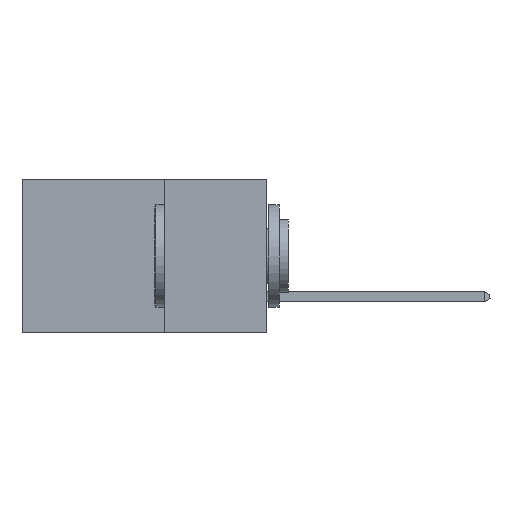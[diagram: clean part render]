
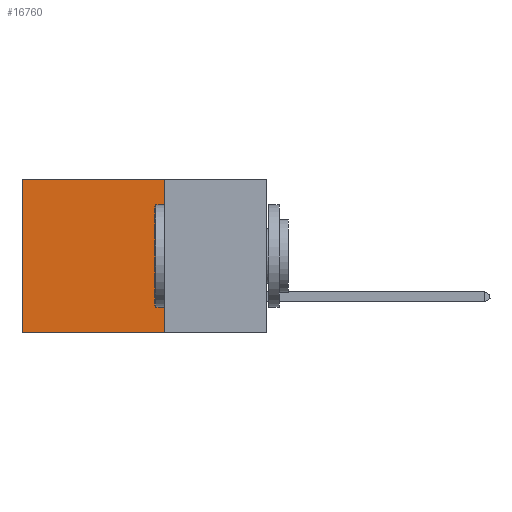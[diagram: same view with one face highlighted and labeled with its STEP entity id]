
A CAD part, left-side view. The second image highlights one B-rep face of the part: STEP entity #16760.
In plain terms, the highlighted planar face has unit normal (-1, 0, 0).
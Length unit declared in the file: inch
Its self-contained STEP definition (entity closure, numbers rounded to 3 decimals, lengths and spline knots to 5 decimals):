
#246 = VERTEX_POINT ( 'NONE', #6477 ) ;
#2128 = VECTOR ( 'NONE', #20580, 39.37008 ) ;
#2588 = PLANE ( 'NONE',  #13594 ) ;
#4701 = LINE ( 'NONE', #8765, #2128 ) ;
#5177 = ORIENTED_EDGE ( 'NONE', *, *, #13428, .F. ) ;
#5771 = CARTESIAN_POINT ( 'NONE',  ( 0.2875, 0.25, -0.375 ) ) ;
#6441 = FACE_OUTER_BOUND ( 'NONE', #14575, .T. ) ;
#6477 = CARTESIAN_POINT ( 'NONE',  ( 0.2875, 0.25, -0.375 ) ) ;
#7086 = CARTESIAN_POINT ( 'NONE',  ( 0.2875, 0.25, -0.375 ) ) ;
#7429 = DIRECTION ( 'NONE',  ( 0., 0., -1. ) ) ;
#8479 = DIRECTION ( 'NONE',  ( 0., 0., -1. ) ) ;
#8746 = EDGE_CURVE ( 'NONE', #13121, #12321, #4701, .T. ) ;
#8765 = CARTESIAN_POINT ( 'NONE',  ( 0.2875, 0.25, 0. ) ) ;
#9564 = LINE ( 'NONE', #10096, #21299 ) ;
#9952 = DIRECTION ( 'NONE',  ( 0., 0., -1. ) ) ;
#10096 = CARTESIAN_POINT ( 'NONE',  ( 0.2875, 0.6, -0.375 ) ) ;
#10702 = ORIENTED_EDGE ( 'NONE', *, *, #16966, .T. ) ;
#10990 = LINE ( 'NONE', #16795, #19336 ) ;
#11635 = VECTOR ( 'NONE', #18829, 39.37008 ) ;
#12037 = EDGE_CURVE ( 'NONE', #246, #14331, #16807, .T. ) ;
#12321 = VERTEX_POINT ( 'NONE', #12616 ) ;
#12616 = CARTESIAN_POINT ( 'NONE',  ( 0.2875, 0.6, 0. ) ) ;
#13121 = VERTEX_POINT ( 'NONE', #19642 ) ;
#13428 = EDGE_CURVE ( 'NONE', #13121, #246, #10990, .T. ) ;
#13594 = AXIS2_PLACEMENT_3D ( 'NONE', #5771, #17560, #7429 ) ;
#14331 = VERTEX_POINT ( 'NONE', #15309 ) ;
#14575 = EDGE_LOOP ( 'NONE', ( #10702, #15559, #5177, #21308 ) ) ;
#15309 = CARTESIAN_POINT ( 'NONE',  ( 0.2875, 0.6, -0.375 ) ) ;
#15559 = ORIENTED_EDGE ( 'NONE', *, *, #12037, .F. ) ;
#16760 = ADVANCED_FACE ( 'NONE', ( #6441 ), #2588, .F. ) ;
#16795 = CARTESIAN_POINT ( 'NONE',  ( 0.2875, 0.25, -0.375 ) ) ;
#16807 = LINE ( 'NONE', #7086, #11635 ) ;
#16966 = EDGE_CURVE ( 'NONE', #12321, #14331, #9564, .T. ) ;
#17560 = DIRECTION ( 'NONE',  ( 1., 0., 0. ) ) ;
#18829 = DIRECTION ( 'NONE',  ( 0., 1., 0. ) ) ;
#19336 = VECTOR ( 'NONE', #8479, 39.37008 ) ;
#19642 = CARTESIAN_POINT ( 'NONE',  ( 0.2875, 0.25, 0. ) ) ;
#20580 = DIRECTION ( 'NONE',  ( 0., 1., 0. ) ) ;
#21299 = VECTOR ( 'NONE', #9952, 39.37008 ) ;
#21308 = ORIENTED_EDGE ( 'NONE', *, *, #8746, .T. ) ;
